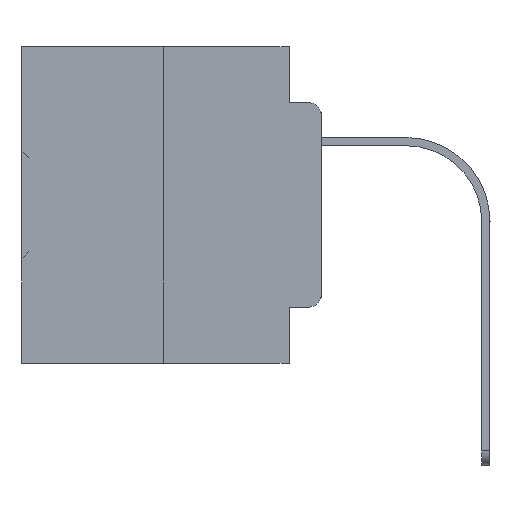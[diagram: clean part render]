
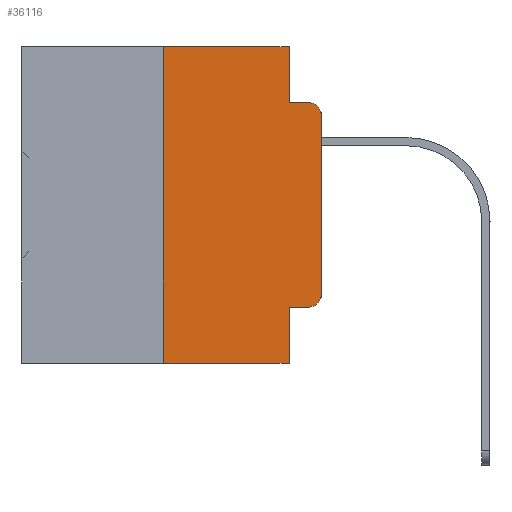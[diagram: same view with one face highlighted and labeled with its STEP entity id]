
A CAD part, left-side view. The second image highlights one B-rep face of the part: STEP entity #36116.
In plain terms, the highlighted planar face has unit normal (-1, 0, 0).
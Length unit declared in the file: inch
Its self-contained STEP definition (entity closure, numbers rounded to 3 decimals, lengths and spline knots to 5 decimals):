
#174 = CARTESIAN_POINT ( 'NONE',  ( 0., 0.473, 0. ) ) ;
#259 = LINE ( 'NONE', #8167, #17273 ) ;
#919 = DIRECTION ( 'NONE',  ( 0., -1., 0. ) ) ;
#1283 = VERTEX_POINT ( 'NONE', #4900 ) ;
#1299 = DIRECTION ( 'NONE',  ( -1., 0., 0. ) ) ;
#1397 = ORIENTED_EDGE ( 'NONE', *, *, #34244, .F. ) ;
#1987 = PLANE ( 'NONE',  #11081 ) ;
#2130 = AXIS2_PLACEMENT_3D ( 'NONE', #23950, #13023, #35488 ) ;
#2896 = CARTESIAN_POINT ( 'NONE',  ( 0., 0.051, 0. ) ) ;
#2962 = CARTESIAN_POINT ( 'NONE',  ( 0., 0.051, -0.4115 ) ) ;
#4207 = DIRECTION ( 'NONE',  ( 0., 0., -1. ) ) ;
#4459 = CIRCLE ( 'NONE', #2130, 0.02 ) ;
#4900 = CARTESIAN_POINT ( 'NONE',  ( 0., 0.25, 0. ) ) ;
#5624 = ORIENTED_EDGE ( 'NONE', *, *, #26403, .T. ) ;
#7835 = FACE_OUTER_BOUND ( 'NONE', #8765, .T. ) ;
#8167 = CARTESIAN_POINT ( 'NONE',  ( 0., 0., 0. ) ) ;
#8574 = VERTEX_POINT ( 'NONE', #14333 ) ;
#8593 = DIRECTION ( 'NONE',  ( 0., -1., 0. ) ) ;
#8765 = EDGE_LOOP ( 'NONE', ( #28894, #15690, #34417, #19495, #12915, #1397, #14924, #29335, #5624, #23634 ) ) ;
#9199 = VERTEX_POINT ( 'NONE', #18652 ) ;
#9234 = CIRCLE ( 'NONE', #9797, 0.02 ) ;
#9378 = VECTOR ( 'NONE', #33126, 39.37008 ) ;
#9797 = AXIS2_PLACEMENT_3D ( 'NONE', #26300, #1299, #4207 ) ;
#10202 = CARTESIAN_POINT ( 'NONE',  ( 0., 0.051, -0.0885 ) ) ;
#11038 = VERTEX_POINT ( 'NONE', #19163 ) ;
#11081 = AXIS2_PLACEMENT_3D ( 'NONE', #13150, #24259, #16267 ) ;
#11222 = VERTEX_POINT ( 'NONE', #27708 ) ;
#11409 = LINE ( 'NONE', #22536, #15961 ) ;
#11978 = EDGE_CURVE ( 'NONE', #20869, #11222, #21988, .T. ) ;
#12077 = CARTESIAN_POINT ( 'NONE',  ( 0., 0.051, -0.4115 ) ) ;
#12915 = ORIENTED_EDGE ( 'NONE', *, *, #28482, .F. ) ;
#13023 = DIRECTION ( 'NONE',  ( -1., 0., 0. ) ) ;
#13150 = CARTESIAN_POINT ( 'NONE',  ( 0., 0.473, 0. ) ) ;
#14143 = EDGE_CURVE ( 'NONE', #11038, #11222, #4459, .T. ) ;
#14196 = CARTESIAN_POINT ( 'NONE',  ( 0., 0.25, -0.5 ) ) ;
#14333 = CARTESIAN_POINT ( 'NONE',  ( 0., 0.02, -0.4115 ) ) ;
#14614 = LINE ( 'NONE', #174, #30190 ) ;
#14924 = ORIENTED_EDGE ( 'NONE', *, *, #35999, .T. ) ;
#15690 = ORIENTED_EDGE ( 'NONE', *, *, #14143, .T. ) ;
#15691 = EDGE_CURVE ( 'NONE', #8574, #9199, #9234, .T. ) ;
#15961 = VECTOR ( 'NONE', #17243, 39.37008 ) ;
#16267 = DIRECTION ( 'NONE',  ( 0., 0., -1. ) ) ;
#16305 = LINE ( 'NONE', #29966, #23751 ) ;
#17243 = DIRECTION ( 'NONE',  ( 0., 0., -1. ) ) ;
#17273 = VECTOR ( 'NONE', #33691, 39.37008 ) ;
#18450 = EDGE_CURVE ( 'NONE', #35576, #28229, #11409, .T. ) ;
#18652 = CARTESIAN_POINT ( 'NONE',  ( 0., 0., -0.3915 ) ) ;
#19031 = DIRECTION ( 'NONE',  ( 0., 0., 1. ) ) ;
#19163 = CARTESIAN_POINT ( 'NONE',  ( 0., 0., -0.1085 ) ) ;
#19495 = ORIENTED_EDGE ( 'NONE', *, *, #33722, .F. ) ;
#20869 = VERTEX_POINT ( 'NONE', #10202 ) ;
#21988 = LINE ( 'NONE', #28157, #9378 ) ;
#22536 = CARTESIAN_POINT ( 'NONE',  ( 0., 0.051, 0. ) ) ;
#23206 = VERTEX_POINT ( 'NONE', #14196 ) ;
#23545 = CARTESIAN_POINT ( 'NONE',  ( 0., 0.051, -0.5 ) ) ;
#23634 = ORIENTED_EDGE ( 'NONE', *, *, #15691, .T. ) ;
#23751 = VECTOR ( 'NONE', #19031, 39.37008 ) ;
#23950 = CARTESIAN_POINT ( 'NONE',  ( 0., 0.02, -0.1085 ) ) ;
#24259 = DIRECTION ( 'NONE',  ( 1., 0., 0. ) ) ;
#24426 = DIRECTION ( 'NONE',  ( 0., 0., -1. ) ) ;
#25326 = CARTESIAN_POINT ( 'NONE',  ( 0., 0.051, 0. ) ) ;
#25745 = LINE ( 'NONE', #12077, #34707 ) ;
#26300 = CARTESIAN_POINT ( 'NONE',  ( 0., 0.02, -0.3915 ) ) ;
#26403 = EDGE_CURVE ( 'NONE', #35576, #8574, #25745, .T. ) ;
#27708 = CARTESIAN_POINT ( 'NONE',  ( 0., 0.02, -0.0885 ) ) ;
#27966 = VECTOR ( 'NONE', #29930, 39.37008 ) ;
#28157 = CARTESIAN_POINT ( 'NONE',  ( 0., 0.051, -0.0885 ) ) ;
#28229 = VERTEX_POINT ( 'NONE', #23545 ) ;
#28482 = EDGE_CURVE ( 'NONE', #1283, #34926, #14614, .T. ) ;
#28810 = EDGE_CURVE ( 'NONE', #9199, #11038, #259, .T. ) ;
#28894 = ORIENTED_EDGE ( 'NONE', *, *, #28810, .T. ) ;
#29335 = ORIENTED_EDGE ( 'NONE', *, *, #18450, .F. ) ;
#29930 = DIRECTION ( 'NONE',  ( 0., -1., 0. ) ) ;
#29966 = CARTESIAN_POINT ( 'NONE',  ( 0., 0.25, 0. ) ) ;
#30124 = CARTESIAN_POINT ( 'NONE',  ( 0., 0.473, -0.5 ) ) ;
#30190 = VECTOR ( 'NONE', #8593, 39.37008 ) ;
#30477 = LINE ( 'NONE', #30124, #27966 ) ;
#33083 = VECTOR ( 'NONE', #24426, 39.37008 ) ;
#33126 = DIRECTION ( 'NONE',  ( 0., -1., 0. ) ) ;
#33540 = LINE ( 'NONE', #2896, #33083 ) ;
#33691 = DIRECTION ( 'NONE',  ( 0., 0., 1. ) ) ;
#33722 = EDGE_CURVE ( 'NONE', #34926, #20869, #33540, .T. ) ;
#34244 = EDGE_CURVE ( 'NONE', #23206, #1283, #16305, .T. ) ;
#34417 = ORIENTED_EDGE ( 'NONE', *, *, #11978, .F. ) ;
#34707 = VECTOR ( 'NONE', #919, 39.37008 ) ;
#34926 = VERTEX_POINT ( 'NONE', #25326 ) ;
#35488 = DIRECTION ( 'NONE',  ( 0., 0., -1. ) ) ;
#35576 = VERTEX_POINT ( 'NONE', #2962 ) ;
#35999 = EDGE_CURVE ( 'NONE', #23206, #28229, #30477, .T. ) ;
#36116 = ADVANCED_FACE ( 'NONE', ( #7835 ), #1987, .F. ) ;
